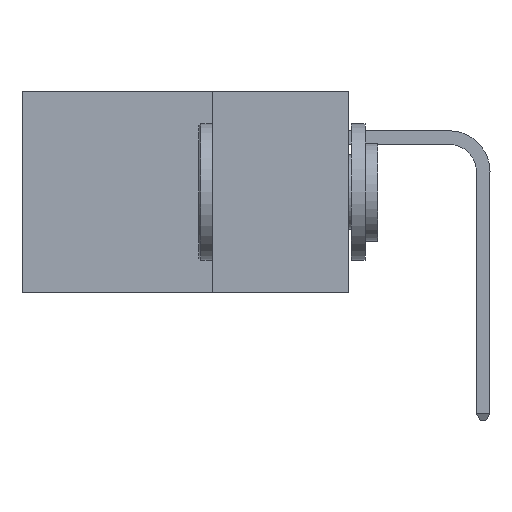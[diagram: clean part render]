
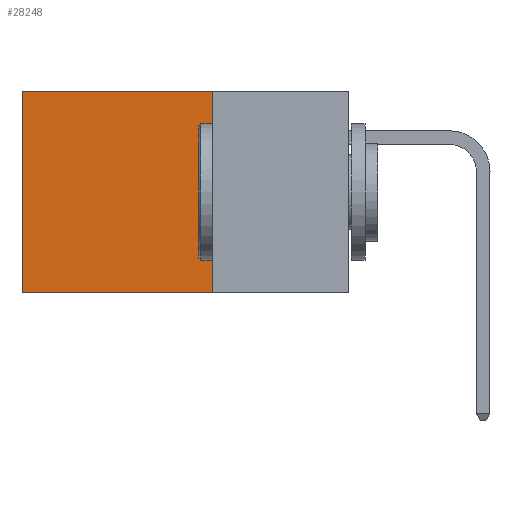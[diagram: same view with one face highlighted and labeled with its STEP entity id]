
A CAD part, left-side view. The second image highlights one B-rep face of the part: STEP entity #28248.
In plain terms, the highlighted planar face has unit normal (-1, 0, 0).
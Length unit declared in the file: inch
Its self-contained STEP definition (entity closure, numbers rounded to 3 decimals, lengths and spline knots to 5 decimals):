
#562 = DIRECTION ( 'NONE',  ( 0., 0., -1. ) ) ;
#1759 = CARTESIAN_POINT ( 'NONE',  ( 0.2875, 0.25, 0. ) ) ;
#2490 = PLANE ( 'NONE',  #28784 ) ;
#2724 = VECTOR ( 'NONE', #6271, 39.37008 ) ;
#3243 = EDGE_CURVE ( 'NONE', #30514, #23956, #19775, .T. ) ;
#5935 = CARTESIAN_POINT ( 'NONE',  ( 0.2875, 0.25, -0.37 ) ) ;
#6271 = DIRECTION ( 'NONE',  ( 0., 0., -1. ) ) ;
#6695 = EDGE_CURVE ( 'NONE', #23956, #15999, #18024, .T. ) ;
#7184 = EDGE_CURVE ( 'NONE', #30514, #19685, #34372, .T. ) ;
#7289 = LINE ( 'NONE', #5935, #35795 ) ;
#8865 = DIRECTION ( 'NONE',  ( 0., 1., 0. ) ) ;
#9193 = CARTESIAN_POINT ( 'NONE',  ( 0.2875, 0.6, 0. ) ) ;
#9971 = CARTESIAN_POINT ( 'NONE',  ( 0.2875, 0.6, -0.37 ) ) ;
#10393 = ORIENTED_EDGE ( 'NONE', *, *, #3243, .T. ) ;
#10457 = DIRECTION ( 'NONE',  ( 0., 1., 0. ) ) ;
#14067 = CARTESIAN_POINT ( 'NONE',  ( 0.2875, 0.25, 0. ) ) ;
#15999 = VERTEX_POINT ( 'NONE', #9971 ) ;
#16964 = DIRECTION ( 'NONE',  ( 0., 0., -1. ) ) ;
#18024 = LINE ( 'NONE', #9193, #2724 ) ;
#18919 = ORIENTED_EDGE ( 'NONE', *, *, #6695, .T. ) ;
#18981 = ORIENTED_EDGE ( 'NONE', *, *, #29006, .F. ) ;
#19152 = CARTESIAN_POINT ( 'NONE',  ( 0.2875, 0.6, 0. ) ) ;
#19685 = VERTEX_POINT ( 'NONE', #34887 ) ;
#19775 = LINE ( 'NONE', #1759, #33026 ) ;
#23893 = FACE_OUTER_BOUND ( 'NONE', #36042, .T. ) ;
#23956 = VERTEX_POINT ( 'NONE', #19152 ) ;
#26205 = CARTESIAN_POINT ( 'NONE',  ( 0.2875, 0.25, 0. ) ) ;
#26835 = VECTOR ( 'NONE', #562, 39.37008 ) ;
#28248 = ADVANCED_FACE ( 'NONE', ( #23893 ), #2490, .F. ) ;
#28784 = AXIS2_PLACEMENT_3D ( 'NONE', #14067, #33932, #16964 ) ;
#29006 = EDGE_CURVE ( 'NONE', #19685, #15999, #7289, .T. ) ;
#29990 = CARTESIAN_POINT ( 'NONE',  ( 0.2875, 0.25, 0. ) ) ;
#30514 = VERTEX_POINT ( 'NONE', #29990 ) ;
#33026 = VECTOR ( 'NONE', #10457, 39.37008 ) ;
#33542 = ORIENTED_EDGE ( 'NONE', *, *, #7184, .F. ) ;
#33932 = DIRECTION ( 'NONE',  ( 1., 0., 0. ) ) ;
#34372 = LINE ( 'NONE', #26205, #26835 ) ;
#34887 = CARTESIAN_POINT ( 'NONE',  ( 0.2875, 0.25, -0.37 ) ) ;
#35795 = VECTOR ( 'NONE', #8865, 39.37008 ) ;
#36042 = EDGE_LOOP ( 'NONE', ( #18919, #18981, #33542, #10393 ) ) ;
